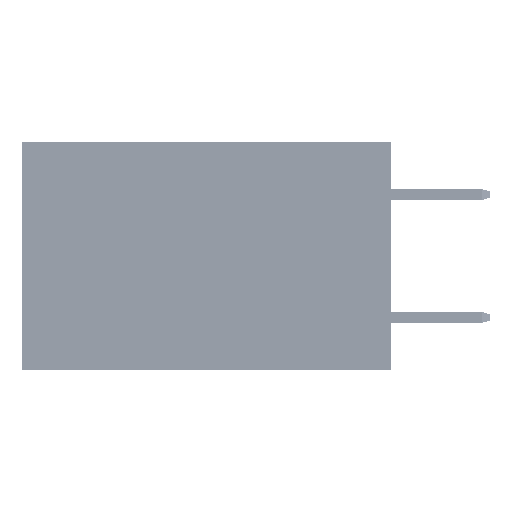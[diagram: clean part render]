
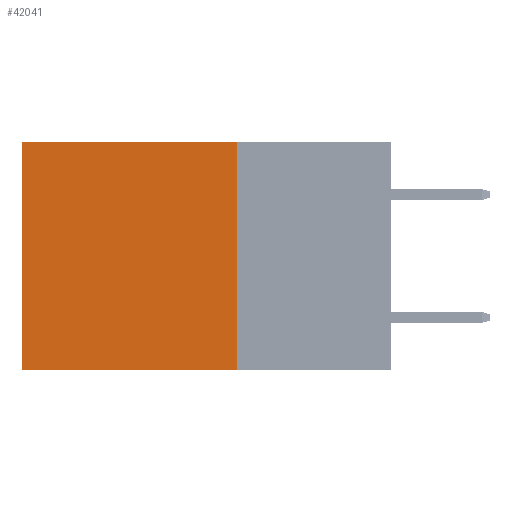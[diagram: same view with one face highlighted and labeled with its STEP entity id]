
A CAD part, left-side view. The second image highlights one B-rep face of the part: STEP entity #42041.
In plain terms, the highlighted planar face has unit normal (-1, 0, 0).
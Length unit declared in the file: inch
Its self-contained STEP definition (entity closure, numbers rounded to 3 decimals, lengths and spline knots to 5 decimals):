
#658 = CARTESIAN_POINT ( 'NONE',  ( 0.2875, 0.6, -0.37 ) ) ;
#836 = VECTOR ( 'NONE', #43741, 39.37008 ) ;
#1846 = CARTESIAN_POINT ( 'NONE',  ( 0.2875, 0.25, 0. ) ) ;
#2224 = CARTESIAN_POINT ( 'NONE',  ( 0.2875, 0.25, 0. ) ) ;
#4082 = EDGE_LOOP ( 'NONE', ( #41772, #45716, #34883, #21811 ) ) ;
#4402 = VERTEX_POINT ( 'NONE', #42827 ) ;
#5076 = DIRECTION ( 'NONE',  ( 0., 1., 0. ) ) ;
#5927 = DIRECTION ( 'NONE',  ( 0., 0., -1. ) ) ;
#14403 = CARTESIAN_POINT ( 'NONE',  ( 0.2875, 0.6, 0. ) ) ;
#16854 = EDGE_CURVE ( 'NONE', #4402, #40729, #30706, .T. ) ;
#17914 = LINE ( 'NONE', #31897, #836 ) ;
#19902 = VERTEX_POINT ( 'NONE', #658 ) ;
#19949 = VECTOR ( 'NONE', #24818, 39.37008 ) ;
#21811 = ORIENTED_EDGE ( 'NONE', *, *, #16854, .T. ) ;
#22663 = EDGE_CURVE ( 'NONE', #40729, #19902, #17914, .T. ) ;
#24818 = DIRECTION ( 'NONE',  ( 0., 1., 0. ) ) ;
#25112 = CARTESIAN_POINT ( 'NONE',  ( 0.2875, 0.25, -0.37 ) ) ;
#26838 = DIRECTION ( 'NONE',  ( 1., 0., 0. ) ) ;
#28422 = EDGE_CURVE ( 'NONE', #4402, #47133, #42343, .T. ) ;
#29209 = CARTESIAN_POINT ( 'NONE',  ( 0.2875, 0.25, 0. ) ) ;
#30189 = LINE ( 'NONE', #25112, #45387 ) ;
#30581 = DIRECTION ( 'NONE',  ( 0., 0., -1. ) ) ;
#30706 = LINE ( 'NONE', #29209, #19949 ) ;
#30994 = EDGE_CURVE ( 'NONE', #47133, #19902, #30189, .T. ) ;
#31897 = CARTESIAN_POINT ( 'NONE',  ( 0.2875, 0.6, 0. ) ) ;
#34883 = ORIENTED_EDGE ( 'NONE', *, *, #28422, .F. ) ;
#35867 = AXIS2_PLACEMENT_3D ( 'NONE', #2224, #26838, #30581 ) ;
#39060 = CARTESIAN_POINT ( 'NONE',  ( 0.2875, 0.25, -0.37 ) ) ;
#40729 = VERTEX_POINT ( 'NONE', #14403 ) ;
#41772 = ORIENTED_EDGE ( 'NONE', *, *, #22663, .T. ) ;
#42041 = ADVANCED_FACE ( 'NONE', ( #50718 ), #46676, .F. ) ;
#42343 = LINE ( 'NONE', #1846, #43008 ) ;
#42827 = CARTESIAN_POINT ( 'NONE',  ( 0.2875, 0.25, 0. ) ) ;
#43008 = VECTOR ( 'NONE', #5927, 39.37008 ) ;
#43741 = DIRECTION ( 'NONE',  ( 0., 0., -1. ) ) ;
#45387 = VECTOR ( 'NONE', #5076, 39.37008 ) ;
#45716 = ORIENTED_EDGE ( 'NONE', *, *, #30994, .F. ) ;
#46676 = PLANE ( 'NONE',  #35867 ) ;
#47133 = VERTEX_POINT ( 'NONE', #39060 ) ;
#50718 = FACE_OUTER_BOUND ( 'NONE', #4082, .T. ) ;
